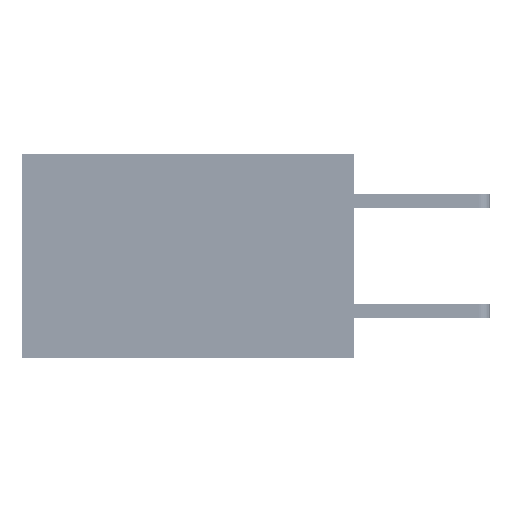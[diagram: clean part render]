
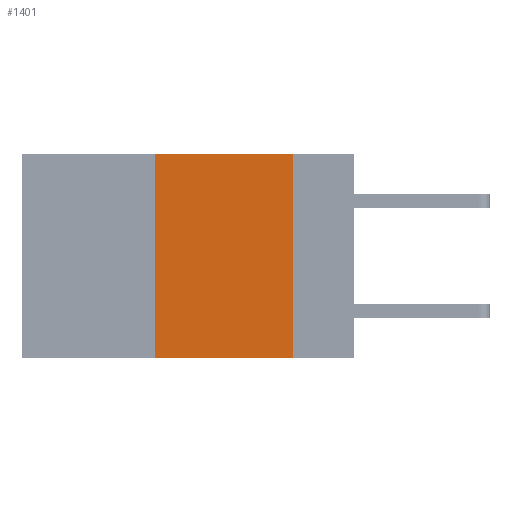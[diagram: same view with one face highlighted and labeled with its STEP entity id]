
A CAD part, left-side view. The second image highlights one B-rep face of the part: STEP entity #1401.
In plain terms, the highlighted planar face has unit normal (-1, 0, 0).
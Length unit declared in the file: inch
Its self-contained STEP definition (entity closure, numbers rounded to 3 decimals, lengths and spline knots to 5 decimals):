
#1036 = VECTOR ( 'NONE', #14695, 39.37008 ) ;
#1401 = ADVANCED_FACE ( 'NONE', ( #1485 ), #3966, .F. ) ;
#1485 = FACE_OUTER_BOUND ( 'NONE', #16688, .T. ) ;
#2938 = DIRECTION ( 'NONE',  ( 0., -1., 0. ) ) ;
#3655 = CARTESIAN_POINT ( 'NONE',  ( 0., 0.36, -0.37 ) ) ;
#3966 = PLANE ( 'NONE',  #6398 ) ;
#6276 = LINE ( 'NONE', #28055, #15611 ) ;
#6398 = AXIS2_PLACEMENT_3D ( 'NONE', #40408, #16837, #39963 ) ;
#7319 = ORIENTED_EDGE ( 'NONE', *, *, #41294, .F. ) ;
#11300 = VERTEX_POINT ( 'NONE', #29249 ) ;
#12084 = CARTESIAN_POINT ( 'NONE',  ( 0., 0.36, 0. ) ) ;
#13979 = LINE ( 'NONE', #28471, #42453 ) ;
#14695 = DIRECTION ( 'NONE',  ( 0., 0., -1. ) ) ;
#15611 = VECTOR ( 'NONE', #2938, 39.37008 ) ;
#16688 = EDGE_LOOP ( 'NONE', ( #34629, #22898, #7319, #29972 ) ) ;
#16837 = DIRECTION ( 'NONE',  ( 1., 0., 0. ) ) ;
#18084 = CARTESIAN_POINT ( 'NONE',  ( 0., 0.6, -0.37 ) ) ;
#22898 = ORIENTED_EDGE ( 'NONE', *, *, #37497, .F. ) ;
#23915 = VECTOR ( 'NONE', #31236, 39.37008 ) ;
#24055 = VERTEX_POINT ( 'NONE', #3655 ) ;
#24281 = CARTESIAN_POINT ( 'NONE',  ( 0., 0.11, 0. ) ) ;
#27351 = EDGE_CURVE ( 'NONE', #24055, #40430, #40986, .T. ) ;
#27673 = CARTESIAN_POINT ( 'NONE',  ( 0., 0.11, -0.37 ) ) ;
#28055 = CARTESIAN_POINT ( 'NONE',  ( 0., 0.6, 0. ) ) ;
#28471 = CARTESIAN_POINT ( 'NONE',  ( 0., 0.36, 0. ) ) ;
#29249 = CARTESIAN_POINT ( 'NONE',  ( 0., 0.11, 0. ) ) ;
#29972 = ORIENTED_EDGE ( 'NONE', *, *, #27351, .T. ) ;
#31236 = DIRECTION ( 'NONE',  ( 0., -1., 0. ) ) ;
#34629 = ORIENTED_EDGE ( 'NONE', *, *, #41838, .F. ) ;
#34702 = DIRECTION ( 'NONE',  ( 0., 0., 1. ) ) ;
#37497 = EDGE_CURVE ( 'NONE', #41971, #11300, #6276, .T. ) ;
#39963 = DIRECTION ( 'NONE',  ( 0., 0., -1. ) ) ;
#40408 = CARTESIAN_POINT ( 'NONE',  ( 0., 0.6, 0. ) ) ;
#40430 = VERTEX_POINT ( 'NONE', #27673 ) ;
#40986 = LINE ( 'NONE', #18084, #23915 ) ;
#41294 = EDGE_CURVE ( 'NONE', #24055, #41971, #13979, .T. ) ;
#41838 = EDGE_CURVE ( 'NONE', #11300, #40430, #42386, .T. ) ;
#41971 = VERTEX_POINT ( 'NONE', #12084 ) ;
#42386 = LINE ( 'NONE', #24281, #1036 ) ;
#42453 = VECTOR ( 'NONE', #34702, 39.37008 ) ;
